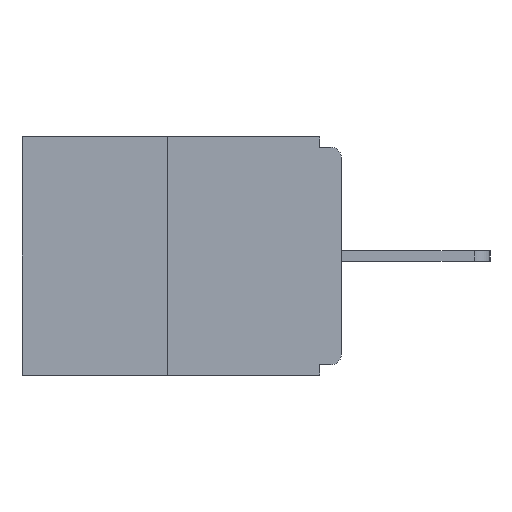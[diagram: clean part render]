
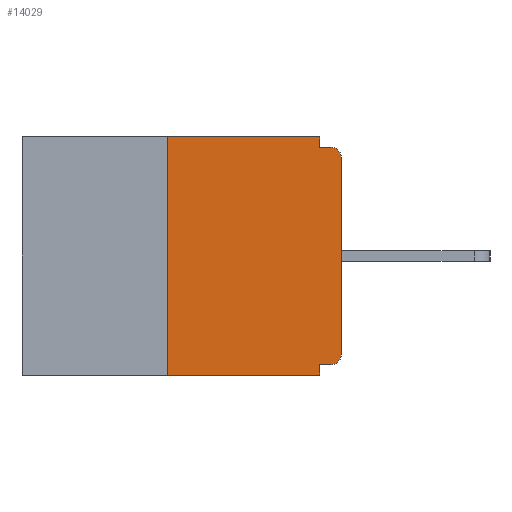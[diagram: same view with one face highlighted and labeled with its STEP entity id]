
A CAD part, left-side view. The second image highlights one B-rep face of the part: STEP entity #14029.
In plain terms, the highlighted planar face has unit normal (-1, 0, 0).
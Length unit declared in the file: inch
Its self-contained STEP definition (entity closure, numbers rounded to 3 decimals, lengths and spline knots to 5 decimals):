
#204 = CARTESIAN_POINT ( 'NONE',  ( 0., 0.46, 0. ) ) ;
#296 = ORIENTED_EDGE ( 'NONE', *, *, #8336, .F. ) ;
#1383 = LINE ( 'NONE', #9797, #10678 ) ;
#2037 = VERTEX_POINT ( 'NONE', #14273 ) ;
#2074 = VERTEX_POINT ( 'NONE', #4823 ) ;
#2114 = LINE ( 'NONE', #13835, #2222 ) ;
#2222 = VECTOR ( 'NONE', #4549, 39.37008 ) ;
#2293 = DIRECTION ( 'NONE',  ( 0., 1., 0. ) ) ;
#2425 = CARTESIAN_POINT ( 'NONE',  ( 0., 0.031, -0.343 ) ) ;
#2479 = PLANE ( 'NONE',  #4790 ) ;
#2506 = DIRECTION ( 'NONE',  ( 0., 0., -1. ) ) ;
#2606 = ORIENTED_EDGE ( 'NONE', *, *, #4691, .F. ) ;
#2617 = CARTESIAN_POINT ( 'NONE',  ( 0., 0.015, -0.03 ) ) ;
#2872 = CARTESIAN_POINT ( 'NONE',  ( 0., 0.031, -0.343 ) ) ;
#3247 = VECTOR ( 'NONE', #2293, 39.37008 ) ;
#3317 = CARTESIAN_POINT ( 'NONE',  ( 0., 0.015, -0.313 ) ) ;
#3455 = EDGE_CURVE ( 'NONE', #6831, #6304, #1383, .T. ) ;
#3634 = EDGE_CURVE ( 'NONE', #14623, #11369, #11810, .T. ) ;
#3805 = CIRCLE ( 'NONE', #12510, 0.015 ) ;
#3845 = ORIENTED_EDGE ( 'NONE', *, *, #3455, .F. ) ;
#4185 = CARTESIAN_POINT ( 'NONE',  ( 0., 0., -0.03 ) ) ;
#4463 = LINE ( 'NONE', #11629, #13372 ) ;
#4549 = DIRECTION ( 'NONE',  ( 0., 0., 1. ) ) ;
#4560 = EDGE_CURVE ( 'NONE', #7851, #6831, #4463, .T. ) ;
#4691 = EDGE_CURVE ( 'NONE', #11369, #7705, #15398, .T. ) ;
#4790 = AXIS2_PLACEMENT_3D ( 'NONE', #10907, #9672, #14437 ) ;
#4823 = CARTESIAN_POINT ( 'NONE',  ( 0., 0., -0.313 ) ) ;
#4894 = LINE ( 'NONE', #204, #9534 ) ;
#4963 = DIRECTION ( 'NONE',  ( 0., -1., 0. ) ) ;
#4984 = FACE_OUTER_BOUND ( 'NONE', #12088, .T. ) ;
#5056 = DIRECTION ( 'NONE',  ( -1., 0., 0. ) ) ;
#5159 = EDGE_CURVE ( 'NONE', #11595, #6304, #14426, .T. ) ;
#5189 = EDGE_CURVE ( 'NONE', #11947, #7705, #14281, .T. ) ;
#5667 = DIRECTION ( 'NONE',  ( -1., 0., 0. ) ) ;
#5693 = CARTESIAN_POINT ( 'NONE',  ( 0., 0.031, 0. ) ) ;
#6303 = VECTOR ( 'NONE', #15272, 39.37008 ) ;
#6304 = VERTEX_POINT ( 'NONE', #8283 ) ;
#6831 = VERTEX_POINT ( 'NONE', #15432 ) ;
#7227 = DIRECTION ( 'NONE',  ( 0., 0., -1. ) ) ;
#7705 = VERTEX_POINT ( 'NONE', #2872 ) ;
#7851 = VERTEX_POINT ( 'NONE', #5693 ) ;
#8283 = CARTESIAN_POINT ( 'NONE',  ( 0., 0.015, -0.015 ) ) ;
#8336 = EDGE_CURVE ( 'NONE', #11947, #2037, #2114, .T. ) ;
#8988 = DIRECTION ( 'NONE',  ( 0., 0., -1. ) ) ;
#9098 = LINE ( 'NONE', #10481, #6303 ) ;
#9534 = VECTOR ( 'NONE', #4963, 39.37008 ) ;
#9672 = DIRECTION ( 'NONE',  ( 1., 0., 0. ) ) ;
#9682 = AXIS2_PLACEMENT_3D ( 'NONE', #2617, #5056, #11981 ) ;
#9797 = CARTESIAN_POINT ( 'NONE',  ( 0., 0., -0.015 ) ) ;
#9804 = DIRECTION ( 'NONE',  ( 0., -1., 0. ) ) ;
#10481 = CARTESIAN_POINT ( 'NONE',  ( 0., 0., 0. ) ) ;
#10626 = VECTOR ( 'NONE', #2506, 39.37008 ) ;
#10678 = VECTOR ( 'NONE', #14586, 39.37008 ) ;
#10907 = CARTESIAN_POINT ( 'NONE',  ( 0., 0.46, 0. ) ) ;
#11369 = VERTEX_POINT ( 'NONE', #12709 ) ;
#11521 = ORIENTED_EDGE ( 'NONE', *, *, #12238, .T. ) ;
#11595 = VERTEX_POINT ( 'NONE', #4185 ) ;
#11605 = ORIENTED_EDGE ( 'NONE', *, *, #5189, .T. ) ;
#11629 = CARTESIAN_POINT ( 'NONE',  ( 0., 0.031, 0. ) ) ;
#11810 = LINE ( 'NONE', #15263, #3247 ) ;
#11947 = VERTEX_POINT ( 'NONE', #13016 ) ;
#11981 = DIRECTION ( 'NONE',  ( 0., 0., -1. ) ) ;
#11999 = ORIENTED_EDGE ( 'NONE', *, *, #13051, .T. ) ;
#12088 = EDGE_LOOP ( 'NONE', ( #13768, #296, #11605, #2606, #14431, #11999, #11521, #13811, #3845, #13323 ) ) ;
#12238 = EDGE_CURVE ( 'NONE', #2074, #11595, #9098, .T. ) ;
#12510 = AXIS2_PLACEMENT_3D ( 'NONE', #3317, #5667, #7227 ) ;
#12665 = VECTOR ( 'NONE', #9804, 39.37008 ) ;
#12709 = CARTESIAN_POINT ( 'NONE',  ( 0., 0.031, -0.328 ) ) ;
#13016 = CARTESIAN_POINT ( 'NONE',  ( 0., 0.25, -0.343 ) ) ;
#13051 = EDGE_CURVE ( 'NONE', #14623, #2074, #3805, .T. ) ;
#13122 = CARTESIAN_POINT ( 'NONE',  ( 0., 0.015, -0.328 ) ) ;
#13323 = ORIENTED_EDGE ( 'NONE', *, *, #4560, .F. ) ;
#13372 = VECTOR ( 'NONE', #8988, 39.37008 ) ;
#13768 = ORIENTED_EDGE ( 'NONE', *, *, #14409, .F. ) ;
#13811 = ORIENTED_EDGE ( 'NONE', *, *, #5159, .T. ) ;
#13835 = CARTESIAN_POINT ( 'NONE',  ( 0., 0.25, 0. ) ) ;
#14029 = ADVANCED_FACE ( 'NONE', ( #4984 ), #2479, .F. ) ;
#14273 = CARTESIAN_POINT ( 'NONE',  ( 0., 0.25, 0. ) ) ;
#14281 = LINE ( 'NONE', #14422, #12665 ) ;
#14409 = EDGE_CURVE ( 'NONE', #2037, #7851, #4894, .T. ) ;
#14422 = CARTESIAN_POINT ( 'NONE',  ( 0., 0.46, -0.343 ) ) ;
#14426 = CIRCLE ( 'NONE', #9682, 0.015 ) ;
#14431 = ORIENTED_EDGE ( 'NONE', *, *, #3634, .F. ) ;
#14437 = DIRECTION ( 'NONE',  ( 0., 0., -1. ) ) ;
#14586 = DIRECTION ( 'NONE',  ( 0., -1., 0. ) ) ;
#14623 = VERTEX_POINT ( 'NONE', #13122 ) ;
#15263 = CARTESIAN_POINT ( 'NONE',  ( 0., 0., -0.328 ) ) ;
#15272 = DIRECTION ( 'NONE',  ( 0., 0., 1. ) ) ;
#15398 = LINE ( 'NONE', #2425, #10626 ) ;
#15432 = CARTESIAN_POINT ( 'NONE',  ( 0., 0.031, -0.015 ) ) ;
